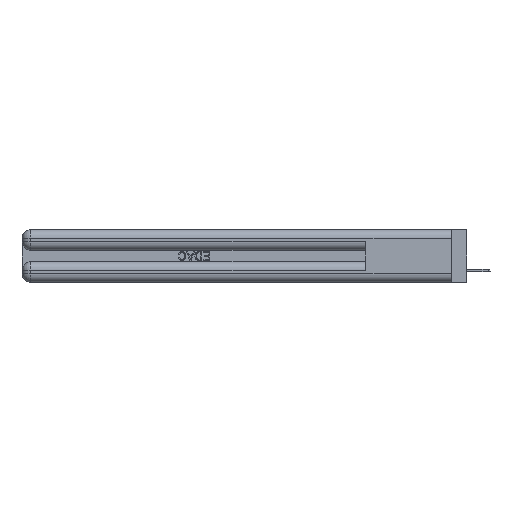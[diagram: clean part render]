
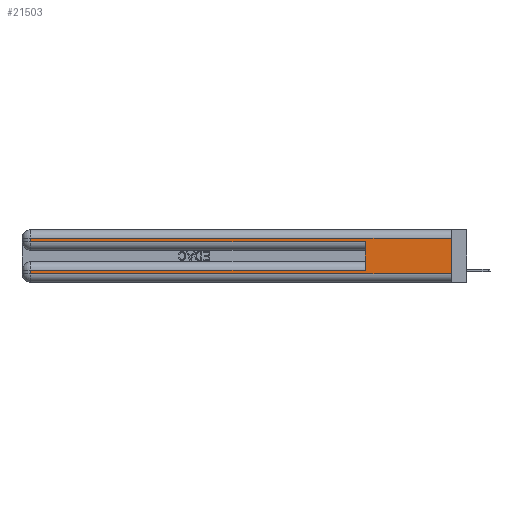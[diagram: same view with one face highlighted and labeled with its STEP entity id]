
A CAD part, left-side view. The second image highlights one B-rep face of the part: STEP entity #21503.
In plain terms, the highlighted planar face has unit normal (-1, 0, 0).
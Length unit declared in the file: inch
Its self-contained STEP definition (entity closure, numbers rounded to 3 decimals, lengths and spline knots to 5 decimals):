
#336 = VERTEX_POINT ( 'NONE', #22187 ) ;
#863 = CARTESIAN_POINT ( 'NONE',  ( 0., 0.6, 0.085 ) ) ;
#941 = LINE ( 'NONE', #16600, #4921 ) ;
#1166 = EDGE_CURVE ( 'NONE', #30184, #26325, #21866, .T. ) ;
#1346 = LINE ( 'NONE', #7591, #25469 ) ;
#2715 = EDGE_LOOP ( 'NONE', ( #10778, #7437, #8459, #29341, #28042, #16123, #33281, #5502 ) ) ;
#3722 = VECTOR ( 'NONE', #25916, 39.37008 ) ;
#4351 = EDGE_CURVE ( 'NONE', #9456, #14588, #32179, .T. ) ;
#4921 = VECTOR ( 'NONE', #36096, 39.37008 ) ;
#5094 = DIRECTION ( 'NONE',  ( 0., -1., 0. ) ) ;
#5502 = ORIENTED_EDGE ( 'NONE', *, *, #17462, .T. ) ;
#5554 = VECTOR ( 'NONE', #12905, 39.37008 ) ;
#7053 = VECTOR ( 'NONE', #12432, 39.37008 ) ;
#7437 = ORIENTED_EDGE ( 'NONE', *, *, #1166, .T. ) ;
#7467 = AXIS2_PLACEMENT_3D ( 'NONE', #11784, #25998, #34092 ) ;
#7510 = EDGE_CURVE ( 'NONE', #26325, #336, #27635, .T. ) ;
#7591 = CARTESIAN_POINT ( 'NONE',  ( 0., 0., 0.06 ) ) ;
#8459 = ORIENTED_EDGE ( 'NONE', *, *, #7510, .T. ) ;
#9456 = VERTEX_POINT ( 'NONE', #863 ) ;
#9460 = DIRECTION ( 'NONE',  ( 0., 0., -1. ) ) ;
#10370 = CARTESIAN_POINT ( 'NONE',  ( 0., 2.94, 0.31 ) ) ;
#10621 = LINE ( 'NONE', #32426, #7053 ) ;
#10665 = CARTESIAN_POINT ( 'NONE',  ( 0., 2.94, 0.085 ) ) ;
#10778 = ORIENTED_EDGE ( 'NONE', *, *, #32977, .F. ) ;
#10797 = FACE_OUTER_BOUND ( 'NONE', #2715, .T. ) ;
#11784 = CARTESIAN_POINT ( 'NONE',  ( 0., 0., 0.37 ) ) ;
#12309 = DIRECTION ( 'NONE',  ( 0., 1., 0. ) ) ;
#12432 = DIRECTION ( 'NONE',  ( 0., -1., 0. ) ) ;
#12905 = DIRECTION ( 'NONE',  ( 0., 1., 0. ) ) ;
#12926 = CARTESIAN_POINT ( 'NONE',  ( 0., 0., 0.31 ) ) ;
#13590 = VECTOR ( 'NONE', #30491, 39.37008 ) ;
#13610 = CARTESIAN_POINT ( 'NONE',  ( 0., 2.94, 0.06 ) ) ;
#14588 = VERTEX_POINT ( 'NONE', #10665 ) ;
#16123 = ORIENTED_EDGE ( 'NONE', *, *, #4351, .T. ) ;
#16243 = LINE ( 'NONE', #18870, #13590 ) ;
#16600 = CARTESIAN_POINT ( 'NONE',  ( 0., 0., 0.37 ) ) ;
#17353 = CARTESIAN_POINT ( 'NONE',  ( 0., 0., 0.31 ) ) ;
#17462 = EDGE_CURVE ( 'NONE', #19009, #22438, #1346, .T. ) ;
#18870 = CARTESIAN_POINT ( 'NONE',  ( 0., 0.6, 0.145 ) ) ;
#19009 = VERTEX_POINT ( 'NONE', #13610 ) ;
#20635 = VECTOR ( 'NONE', #9460, 39.37008 ) ;
#20762 = EDGE_CURVE ( 'NONE', #14588, #19009, #34034, .T. ) ;
#20896 = CARTESIAN_POINT ( 'NONE',  ( 0., 0., 0.085 ) ) ;
#21503 = ADVANCED_FACE ( 'NONE', ( #10797 ), #28800, .F. ) ;
#21866 = LINE ( 'NONE', #17353, #5554 ) ;
#22187 = CARTESIAN_POINT ( 'NONE',  ( 0., 2.94, 0.285 ) ) ;
#22438 = VERTEX_POINT ( 'NONE', #35796 ) ;
#23734 = CARTESIAN_POINT ( 'NONE',  ( 0., 0.6, 0.285 ) ) ;
#23883 = EDGE_CURVE ( 'NONE', #9456, #26183, #16243, .T. ) ;
#25469 = VECTOR ( 'NONE', #5094, 39.37008 ) ;
#25916 = DIRECTION ( 'NONE',  ( 0., 0., -1. ) ) ;
#25998 = DIRECTION ( 'NONE',  ( 1., 0., 0. ) ) ;
#26183 = VERTEX_POINT ( 'NONE', #23734 ) ;
#26244 = CARTESIAN_POINT ( 'NONE',  ( 0., 2.94, 0.37 ) ) ;
#26325 = VERTEX_POINT ( 'NONE', #10370 ) ;
#27635 = LINE ( 'NONE', #26244, #20635 ) ;
#28042 = ORIENTED_EDGE ( 'NONE', *, *, #23883, .F. ) ;
#28800 = PLANE ( 'NONE',  #7467 ) ;
#29341 = ORIENTED_EDGE ( 'NONE', *, *, #33885, .T. ) ;
#30184 = VERTEX_POINT ( 'NONE', #12926 ) ;
#30491 = DIRECTION ( 'NONE',  ( 0., 0., 1. ) ) ;
#31572 = CARTESIAN_POINT ( 'NONE',  ( 0., 2.94, 0.37 ) ) ;
#32179 = LINE ( 'NONE', #20896, #34820 ) ;
#32426 = CARTESIAN_POINT ( 'NONE',  ( 0., 0., 0.285 ) ) ;
#32977 = EDGE_CURVE ( 'NONE', #30184, #22438, #941, .T. ) ;
#33281 = ORIENTED_EDGE ( 'NONE', *, *, #20762, .T. ) ;
#33885 = EDGE_CURVE ( 'NONE', #336, #26183, #10621, .T. ) ;
#34034 = LINE ( 'NONE', #31572, #3722 ) ;
#34092 = DIRECTION ( 'NONE',  ( 0., 0., -1. ) ) ;
#34820 = VECTOR ( 'NONE', #12309, 39.37008 ) ;
#35796 = CARTESIAN_POINT ( 'NONE',  ( 0., 0., 0.06 ) ) ;
#36096 = DIRECTION ( 'NONE',  ( 0., 0., -1. ) ) ;
